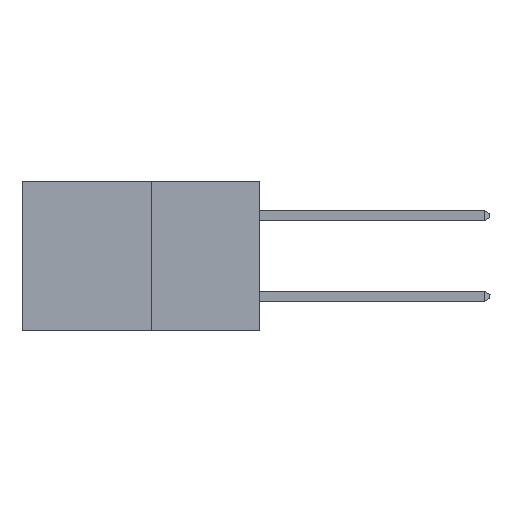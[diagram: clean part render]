
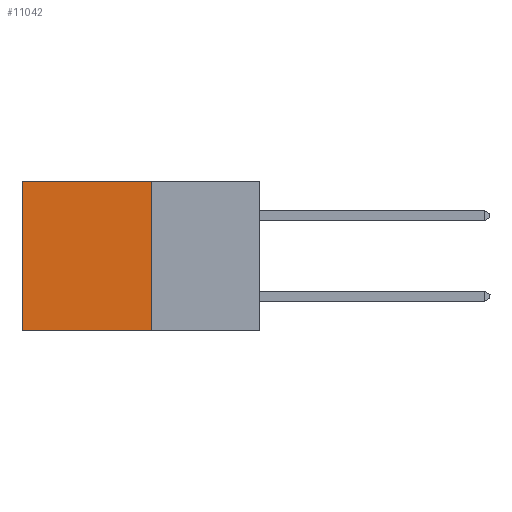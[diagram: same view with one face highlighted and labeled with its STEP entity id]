
A CAD part, left-side view. The second image highlights one B-rep face of the part: STEP entity #11042.
In plain terms, the highlighted planar face has unit normal (-1, 0, 0).
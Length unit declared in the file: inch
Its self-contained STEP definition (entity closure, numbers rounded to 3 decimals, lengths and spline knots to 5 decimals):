
#2111 = CARTESIAN_POINT ( 'NONE',  ( 0.277, 0.27, -0.37 ) ) ;
#2337 = EDGE_LOOP ( 'NONE', ( #11469, #22702, #9031, #14193 ) ) ;
#3622 = PLANE ( 'NONE',  #18024 ) ;
#6143 = CARTESIAN_POINT ( 'NONE',  ( 0.277, 0.27, 0. ) ) ;
#6150 = VECTOR ( 'NONE', #11886, 39.37008 ) ;
#6169 = DIRECTION ( 'NONE',  ( 1., 0., 0. ) ) ;
#7183 = CARTESIAN_POINT ( 'NONE',  ( 0.277, 0.27, -0.37 ) ) ;
#7359 = EDGE_CURVE ( 'NONE', #16324, #12201, #21696, .T. ) ;
#7363 = DIRECTION ( 'NONE',  ( 0., 0., -1. ) ) ;
#7590 = DIRECTION ( 'NONE',  ( 0., 1., 0. ) ) ;
#8417 = VECTOR ( 'NONE', #7363, 39.37008 ) ;
#9031 = ORIENTED_EDGE ( 'NONE', *, *, #29408, .F. ) ;
#11042 = ADVANCED_FACE ( 'NONE', ( #12237 ), #3622, .F. ) ;
#11469 = ORIENTED_EDGE ( 'NONE', *, *, #15681, .T. ) ;
#11835 = CARTESIAN_POINT ( 'NONE',  ( 0.277, 0.27, -0.37 ) ) ;
#11886 = DIRECTION ( 'NONE',  ( 0., 1., 0. ) ) ;
#12201 = VERTEX_POINT ( 'NONE', #26643 ) ;
#12237 = FACE_OUTER_BOUND ( 'NONE', #2337, .T. ) ;
#13672 = LINE ( 'NONE', #19348, #6150 ) ;
#14193 = ORIENTED_EDGE ( 'NONE', *, *, #17602, .T. ) ;
#14962 = CARTESIAN_POINT ( 'NONE',  ( 0.277, 0.59, -0.37 ) ) ;
#15681 = EDGE_CURVE ( 'NONE', #26115, #12201, #28922, .T. ) ;
#16324 = VERTEX_POINT ( 'NONE', #2111 ) ;
#17602 = EDGE_CURVE ( 'NONE', #23311, #26115, #13672, .T. ) ;
#18024 = AXIS2_PLACEMENT_3D ( 'NONE', #21156, #6169, #23608 ) ;
#19348 = CARTESIAN_POINT ( 'NONE',  ( 0.277, 0.27, 0. ) ) ;
#20095 = CARTESIAN_POINT ( 'NONE',  ( 0.277, 0.59, 0. ) ) ;
#20931 = VECTOR ( 'NONE', #7590, 39.37008 ) ;
#21156 = CARTESIAN_POINT ( 'NONE',  ( 0.277, 0.27, -0.37 ) ) ;
#21696 = LINE ( 'NONE', #7183, #20931 ) ;
#22465 = VECTOR ( 'NONE', #24158, 39.37008 ) ;
#22702 = ORIENTED_EDGE ( 'NONE', *, *, #7359, .F. ) ;
#23252 = LINE ( 'NONE', #11835, #22465 ) ;
#23311 = VERTEX_POINT ( 'NONE', #6143 ) ;
#23608 = DIRECTION ( 'NONE',  ( 0., 0., -1. ) ) ;
#24158 = DIRECTION ( 'NONE',  ( 0., 0., -1. ) ) ;
#26115 = VERTEX_POINT ( 'NONE', #20095 ) ;
#26643 = CARTESIAN_POINT ( 'NONE',  ( 0.277, 0.59, -0.37 ) ) ;
#28922 = LINE ( 'NONE', #14962, #8417 ) ;
#29408 = EDGE_CURVE ( 'NONE', #23311, #16324, #23252, .T. ) ;
